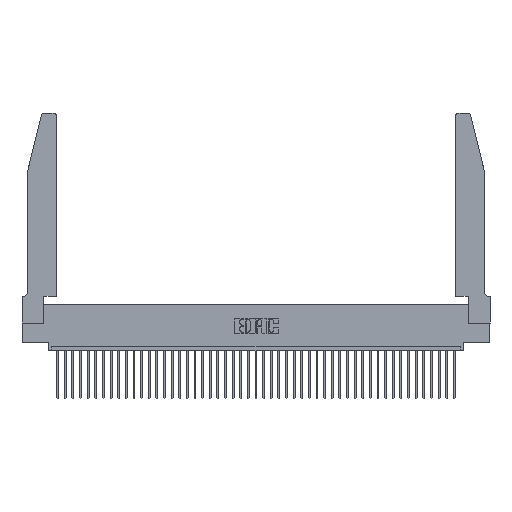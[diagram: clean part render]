
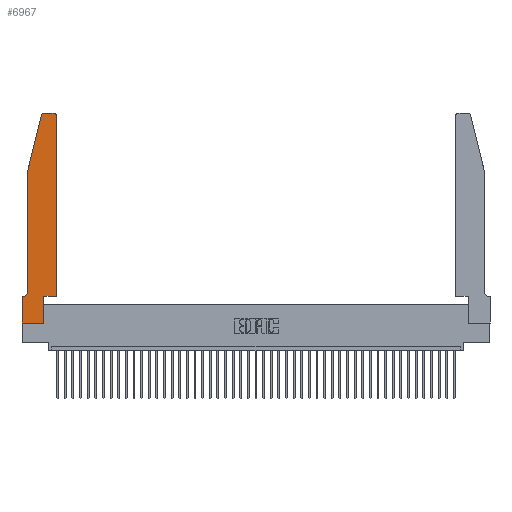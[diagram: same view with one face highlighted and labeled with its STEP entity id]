
A CAD part, top view. The second image highlights one B-rep face of the part: STEP entity #6967.
In plain terms, the highlighted planar face has unit normal (0, 0, 1).
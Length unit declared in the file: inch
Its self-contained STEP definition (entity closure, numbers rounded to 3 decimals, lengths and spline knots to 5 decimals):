
#684 = LINE ( 'NONE', #27203, #12814 ) ;
#1164 = LINE ( 'NONE', #8152, #4924 ) ;
#1253 = DIRECTION ( 'NONE',  ( 0., 0., 1. ) ) ;
#1286 = ORIENTED_EDGE ( 'NONE', *, *, #19658, .T. ) ;
#1314 = CARTESIAN_POINT ( 'NONE',  ( 0.4505, 0.35, 0.37 ) ) ;
#1797 = AXIS2_PLACEMENT_3D ( 'NONE', #40547, #7173, #7581 ) ;
#1961 = DIRECTION ( 'NONE',  ( 0., 0., 1. ) ) ;
#2119 = LINE ( 'NONE', #13710, #22527 ) ;
#3438 = EDGE_CURVE ( 'NONE', #36495, #42077, #684, .T. ) ;
#3607 = CARTESIAN_POINT ( 'NONE',  ( 0.2605, 2.75, 0.37 ) ) ;
#4924 = VECTOR ( 'NONE', #24929, 39.37008 ) ;
#5096 = CARTESIAN_POINT ( 'NONE',  ( 0.2865, 0.35, 0.37 ) ) ;
#5340 = CARTESIAN_POINT ( 'NONE',  ( 0.0755, 0.35, 0.37 ) ) ;
#5658 = DIRECTION ( 'NONE',  ( 1., 0., 0. ) ) ;
#6258 = CARTESIAN_POINT ( 'NONE',  ( 0.0055, 0.35, 0.37 ) ) ;
#6889 = DIRECTION ( 'NONE',  ( -1., 0., 0. ) ) ;
#6967 = ADVANCED_FACE ( 'NONE', ( #40692 ), #34327, .T. ) ;
#7173 = DIRECTION ( 'NONE',  ( 0., 0., 1. ) ) ;
#7581 = DIRECTION ( 'NONE',  ( 1., 0., 0. ) ) ;
#7761 = EDGE_CURVE ( 'NONE', #8158, #31373, #37958, .T. ) ;
#7836 = LINE ( 'NONE', #25299, #40749 ) ;
#8152 = CARTESIAN_POINT ( 'NONE',  ( 0.4505, 0.35, 0.37 ) ) ;
#8158 = VERTEX_POINT ( 'NONE', #28815 ) ;
#8176 = LINE ( 'NONE', #8906, #19729 ) ;
#8906 = CARTESIAN_POINT ( 'NONE',  ( 0.2865, 0.35, 0.37 ) ) ;
#9370 = DIRECTION ( 'NONE',  ( 0., 0., -1. ) ) ;
#10406 = EDGE_CURVE ( 'NONE', #42077, #42462, #23650, .T. ) ;
#10862 = VERTEX_POINT ( 'NONE', #36515 ) ;
#11382 = LINE ( 'NONE', #5340, #31671 ) ;
#11572 = VERTEX_POINT ( 'NONE', #13738 ) ;
#12416 = ORIENTED_EDGE ( 'NONE', *, *, #15174, .T. ) ;
#12814 = VECTOR ( 'NONE', #33719, 39.37008 ) ;
#12957 = EDGE_LOOP ( 'NONE', ( #29387, #22074, #16858, #14566, #24696, #1286, #25761, #34670, #28649, #37369, #12416, #35217 ) ) ;
#13592 = CARTESIAN_POINT ( 'NONE',  ( 0.0755, 0.42, 0.37 ) ) ;
#13710 = CARTESIAN_POINT ( 'NONE',  ( 0.0755, 2., 0.37 ) ) ;
#13738 = CARTESIAN_POINT ( 'NONE',  ( 0.2865, 0., 0.37 ) ) ;
#13928 = VECTOR ( 'NONE', #5658, 39.37008 ) ;
#13985 = VECTOR ( 'NONE', #6889, 39.37008 ) ;
#14566 = ORIENTED_EDGE ( 'NONE', *, *, #3438, .T. ) ;
#15174 = EDGE_CURVE ( 'NONE', #36690, #33031, #1164, .T. ) ;
#15374 = DIRECTION ( 'NONE',  ( 1., 0., 0. ) ) ;
#15927 = CARTESIAN_POINT ( 'NONE',  ( 0.0755, 2., 0.37 ) ) ;
#16076 = CARTESIAN_POINT ( 'NONE',  ( 0.284, 2.75, 0.37 ) ) ;
#16858 = ORIENTED_EDGE ( 'NONE', *, *, #31017, .T. ) ;
#17483 = EDGE_CURVE ( 'NONE', #24957, #36690, #7836, .T. ) ;
#17782 = VERTEX_POINT ( 'NONE', #19766 ) ;
#18710 = DIRECTION ( 'NONE',  ( 1., 0., 0. ) ) ;
#19658 = EDGE_CURVE ( 'NONE', #42462, #10862, #11382, .T. ) ;
#19729 = VECTOR ( 'NONE', #19886, 39.37008 ) ;
#19766 = CARTESIAN_POINT ( 'NONE',  ( 0.25487, 2.72718, 0.37 ) ) ;
#19886 = DIRECTION ( 'NONE',  ( 0., 1., 0. ) ) ;
#20752 = CARTESIAN_POINT ( 'NONE',  ( 0., 0., 0.37 ) ) ;
#22031 = CARTESIAN_POINT ( 'NONE',  ( 0.4205, 2.72, 0.37 ) ) ;
#22074 = ORIENTED_EDGE ( 'NONE', *, *, #32623, .T. ) ;
#22527 = VECTOR ( 'NONE', #40385, 39.37008 ) ;
#23279 = DIRECTION ( 'NONE',  ( 0., -1., 0. ) ) ;
#23559 = CARTESIAN_POINT ( 'NONE',  ( 0., 0., 0.37 ) ) ;
#23628 = CARTESIAN_POINT ( 'NONE',  ( 0.4505, 2.72, 0.37 ) ) ;
#23650 = CIRCLE ( 'NONE', #37418, 0.07 ) ;
#24696 = ORIENTED_EDGE ( 'NONE', *, *, #10406, .T. ) ;
#24929 = DIRECTION ( 'NONE',  ( 0., 1., 0. ) ) ;
#24957 = VERTEX_POINT ( 'NONE', #5096 ) ;
#25284 = DIRECTION ( 'NONE',  ( 1., 0., 0. ) ) ;
#25299 = CARTESIAN_POINT ( 'NONE',  ( 0.4505, 0.35, 0.37 ) ) ;
#25761 = ORIENTED_EDGE ( 'NONE', *, *, #40269, .T. ) ;
#26219 = DIRECTION ( 'NONE',  ( -1., 0., 0. ) ) ;
#27203 = CARTESIAN_POINT ( 'NONE',  ( 0.0755, 2., 0.37 ) ) ;
#28649 = ORIENTED_EDGE ( 'NONE', *, *, #41924, .T. ) ;
#28815 = CARTESIAN_POINT ( 'NONE',  ( 0.4205, 2.75, 0.37 ) ) ;
#29387 = ORIENTED_EDGE ( 'NONE', *, *, #7761, .T. ) ;
#31017 = EDGE_CURVE ( 'NONE', #17782, #36495, #2119, .T. ) ;
#31373 = VERTEX_POINT ( 'NONE', #16076 ) ;
#31591 = LINE ( 'NONE', #42731, #13928 ) ;
#31671 = VECTOR ( 'NONE', #26219, 39.37008 ) ;
#32579 = CIRCLE ( 'NONE', #37318, 0.03 ) ;
#32623 = EDGE_CURVE ( 'NONE', #31373, #17782, #32579, .T. ) ;
#33031 = VERTEX_POINT ( 'NONE', #23628 ) ;
#33719 = DIRECTION ( 'NONE',  ( 0., -1., 0. ) ) ;
#34224 = VERTEX_POINT ( 'NONE', #20752 ) ;
#34327 = PLANE ( 'NONE',  #1797 ) ;
#34670 = ORIENTED_EDGE ( 'NONE', *, *, #42424, .T. ) ;
#35217 = ORIENTED_EDGE ( 'NONE', *, *, #41696, .T. ) ;
#36010 = DIRECTION ( 'NONE',  ( -1., 0., 0. ) ) ;
#36495 = VERTEX_POINT ( 'NONE', #15927 ) ;
#36515 = CARTESIAN_POINT ( 'NONE',  ( 0., 0.35, 0.37 ) ) ;
#36690 = VERTEX_POINT ( 'NONE', #1314 ) ;
#37318 = AXIS2_PLACEMENT_3D ( 'NONE', #41474, #1253, #25284 ) ;
#37369 = ORIENTED_EDGE ( 'NONE', *, *, #17483, .T. ) ;
#37418 = AXIS2_PLACEMENT_3D ( 'NONE', #42790, #9370, #36010 ) ;
#37958 = LINE ( 'NONE', #3607, #13985 ) ;
#38060 = VECTOR ( 'NONE', #23279, 39.37008 ) ;
#39147 = LINE ( 'NONE', #23559, #38060 ) ;
#40269 = EDGE_CURVE ( 'NONE', #10862, #34224, #39147, .T. ) ;
#40376 = AXIS2_PLACEMENT_3D ( 'NONE', #22031, #1961, #18710 ) ;
#40385 = DIRECTION ( 'NONE',  ( -0.239, -0.971, 0. ) ) ;
#40547 = CARTESIAN_POINT ( 'NONE',  ( 0., 0.35, 0.37 ) ) ;
#40692 = FACE_OUTER_BOUND ( 'NONE', #12957, .T. ) ;
#40749 = VECTOR ( 'NONE', #15374, 39.37008 ) ;
#41474 = CARTESIAN_POINT ( 'NONE',  ( 0.284, 2.72, 0.37 ) ) ;
#41632 = CIRCLE ( 'NONE', #40376, 0.03 ) ;
#41696 = EDGE_CURVE ( 'NONE', #33031, #8158, #41632, .T. ) ;
#41924 = EDGE_CURVE ( 'NONE', #11572, #24957, #8176, .T. ) ;
#42077 = VERTEX_POINT ( 'NONE', #13592 ) ;
#42424 = EDGE_CURVE ( 'NONE', #34224, #11572, #31591, .T. ) ;
#42462 = VERTEX_POINT ( 'NONE', #6258 ) ;
#42731 = CARTESIAN_POINT ( 'NONE',  ( 0., 0., 0.37 ) ) ;
#42790 = CARTESIAN_POINT ( 'NONE',  ( 0.0055, 0.42, 0.37 ) ) ;
